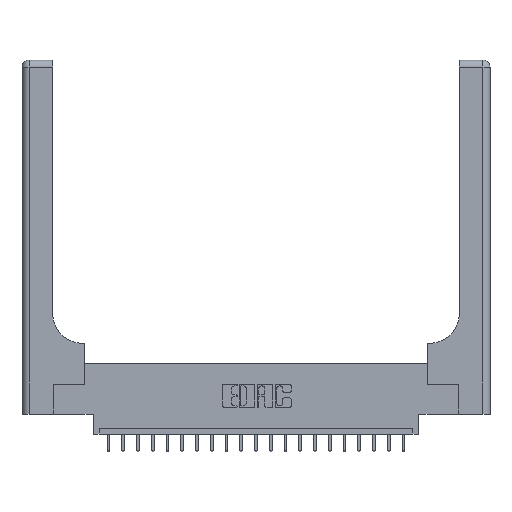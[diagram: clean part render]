
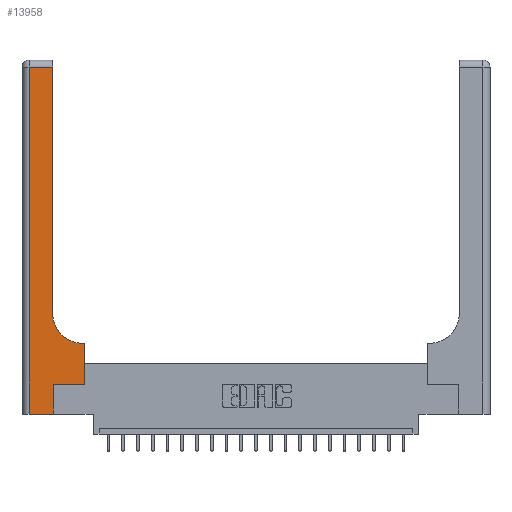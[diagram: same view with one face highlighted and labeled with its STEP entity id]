
A CAD part, top view. The second image highlights one B-rep face of the part: STEP entity #13958.
In plain terms, the highlighted planar face has unit normal (0, 0, 1).
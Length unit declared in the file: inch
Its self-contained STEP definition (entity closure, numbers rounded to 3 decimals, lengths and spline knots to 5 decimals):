
#3 = LINE ( 'NONE', #20273, #2064 ) ;
#542 = DIRECTION ( 'NONE',  ( 1., 0., 0. ) ) ;
#676 = VERTEX_POINT ( 'NONE', #12682 ) ;
#1202 = LINE ( 'NONE', #15344, #6350 ) ;
#1246 = CARTESIAN_POINT ( 'NONE',  ( 0.528, 0.25, 0.37 ) ) ;
#1527 = VECTOR ( 'NONE', #18745, 39.37008 ) ;
#1591 = CARTESIAN_POINT ( 'NONE',  ( 0.265, 0., 0.37 ) ) ;
#2064 = VECTOR ( 'NONE', #7356, 39.37008 ) ;
#2076 = EDGE_CURVE ( 'NONE', #12778, #6023, #13421, .T. ) ;
#3259 = EDGE_CURVE ( 'NONE', #17150, #12778, #16829, .T. ) ;
#4465 = ORIENTED_EDGE ( 'NONE', *, *, #20351, .T. ) ;
#5524 = CARTESIAN_POINT ( 'NONE',  ( 0.26, 0.6, 0.37 ) ) ;
#5667 = CIRCLE ( 'NONE', #9579, 0.25 ) ;
#6023 = VERTEX_POINT ( 'NONE', #11790 ) ;
#6214 = PLANE ( 'NONE',  #12995 ) ;
#6225 = VECTOR ( 'NONE', #11036, 39.37008 ) ;
#6350 = VECTOR ( 'NONE', #20191, 39.37008 ) ;
#6503 = CARTESIAN_POINT ( 'NONE',  ( 0.26, 0.85, 0.37 ) ) ;
#6587 = CARTESIAN_POINT ( 'NONE',  ( 0.528, 0.25, 0.37 ) ) ;
#7141 = CARTESIAN_POINT ( 'NONE',  ( 0., 0., 0.37 ) ) ;
#7356 = DIRECTION ( 'NONE',  ( 0., 1., 0. ) ) ;
#7526 = EDGE_CURVE ( 'NONE', #17454, #16370, #9513, .T. ) ;
#7780 = EDGE_CURVE ( 'NONE', #16926, #676, #3, .T. ) ;
#7928 = DIRECTION ( 'NONE',  ( -1., 0., 0. ) ) ;
#8538 = DIRECTION ( 'NONE',  ( 1., 0., 0. ) ) ;
#9007 = ORIENTED_EDGE ( 'NONE', *, *, #14771, .T. ) ;
#9076 = VECTOR ( 'NONE', #14671, 39.37008 ) ;
#9513 = LINE ( 'NONE', #6587, #15411 ) ;
#9579 = AXIS2_PLACEMENT_3D ( 'NONE', #10101, #18043, #8538 ) ;
#9621 = CARTESIAN_POINT ( 'NONE',  ( 0.265, 0.25, 0.37 ) ) ;
#9794 = CARTESIAN_POINT ( 'NONE',  ( 0.528, 0.6, 0.37 ) ) ;
#10101 = CARTESIAN_POINT ( 'NONE',  ( 0.51, 0.85, 0.37 ) ) ;
#11036 = DIRECTION ( 'NONE',  ( -1., 0., 0. ) ) ;
#11292 = LINE ( 'NONE', #9621, #12083 ) ;
#11451 = VECTOR ( 'NONE', #542, 39.37008 ) ;
#11790 = CARTESIAN_POINT ( 'NONE',  ( 0.265, 0.25, 0.37 ) ) ;
#11821 = EDGE_CURVE ( 'NONE', #13370, #17150, #1202, .T. ) ;
#11852 = LINE ( 'NONE', #14255, #6225 ) ;
#12083 = VECTOR ( 'NONE', #16215, 39.37008 ) ;
#12464 = CARTESIAN_POINT ( 'NONE',  ( 0.06, 2.94, 0.37 ) ) ;
#12682 = CARTESIAN_POINT ( 'NONE',  ( 0.26, 2.94, 0.37 ) ) ;
#12778 = VERTEX_POINT ( 'NONE', #1591 ) ;
#12995 = AXIS2_PLACEMENT_3D ( 'NONE', #17706, #21129, #7928 ) ;
#13221 = DIRECTION ( 'NONE',  ( 0., 1., 0. ) ) ;
#13370 = VERTEX_POINT ( 'NONE', #12464 ) ;
#13421 = LINE ( 'NONE', #19658, #9076 ) ;
#13958 = ADVANCED_FACE ( 'NONE', ( #20544 ), #6214, .F. ) ;
#14041 = ORIENTED_EDGE ( 'NONE', *, *, #7526, .T. ) ;
#14255 = CARTESIAN_POINT ( 'NONE',  ( 0., 2.94, 0.37 ) ) ;
#14671 = DIRECTION ( 'NONE',  ( 0., 1., 0. ) ) ;
#14736 = EDGE_CURVE ( 'NONE', #6023, #17454, #11292, .T. ) ;
#14771 = EDGE_CURVE ( 'NONE', #19750, #16926, #5667, .T. ) ;
#15344 = CARTESIAN_POINT ( 'NONE',  ( 0.06, 3., 0.37 ) ) ;
#15411 = VECTOR ( 'NONE', #13221, 39.37008 ) ;
#15681 = ORIENTED_EDGE ( 'NONE', *, *, #11821, .T. ) ;
#15795 = ORIENTED_EDGE ( 'NONE', *, *, #3259, .T. ) ;
#15960 = EDGE_CURVE ( 'NONE', #16370, #19750, #16884, .T. ) ;
#16215 = DIRECTION ( 'NONE',  ( 1., 0., 0. ) ) ;
#16252 = ORIENTED_EDGE ( 'NONE', *, *, #14736, .T. ) ;
#16370 = VERTEX_POINT ( 'NONE', #9794 ) ;
#16829 = LINE ( 'NONE', #7141, #11451 ) ;
#16884 = LINE ( 'NONE', #5524, #1527 ) ;
#16926 = VERTEX_POINT ( 'NONE', #6503 ) ;
#17150 = VERTEX_POINT ( 'NONE', #20266 ) ;
#17454 = VERTEX_POINT ( 'NONE', #1246 ) ;
#17619 = ORIENTED_EDGE ( 'NONE', *, *, #7780, .T. ) ;
#17706 = CARTESIAN_POINT ( 'NONE',  ( 0., 3., 0.37 ) ) ;
#18043 = DIRECTION ( 'NONE',  ( 0., 0., -1. ) ) ;
#18354 = EDGE_LOOP ( 'NONE', ( #17619, #4465, #15681, #15795, #20714, #16252, #14041, #19607, #9007 ) ) ;
#18745 = DIRECTION ( 'NONE',  ( -1., 0., 0. ) ) ;
#18999 = CARTESIAN_POINT ( 'NONE',  ( 0.51, 0.6, 0.37 ) ) ;
#19607 = ORIENTED_EDGE ( 'NONE', *, *, #15960, .T. ) ;
#19658 = CARTESIAN_POINT ( 'NONE',  ( 0.265, 0., 0.37 ) ) ;
#19750 = VERTEX_POINT ( 'NONE', #18999 ) ;
#20191 = DIRECTION ( 'NONE',  ( 0., -1., 0. ) ) ;
#20266 = CARTESIAN_POINT ( 'NONE',  ( 0.06, 0., 0.37 ) ) ;
#20273 = CARTESIAN_POINT ( 'NONE',  ( 0.26, 3., 0.37 ) ) ;
#20351 = EDGE_CURVE ( 'NONE', #676, #13370, #11852, .T. ) ;
#20544 = FACE_OUTER_BOUND ( 'NONE', #18354, .T. ) ;
#20714 = ORIENTED_EDGE ( 'NONE', *, *, #2076, .T. ) ;
#21129 = DIRECTION ( 'NONE',  ( 0., 0., -1. ) ) ;
